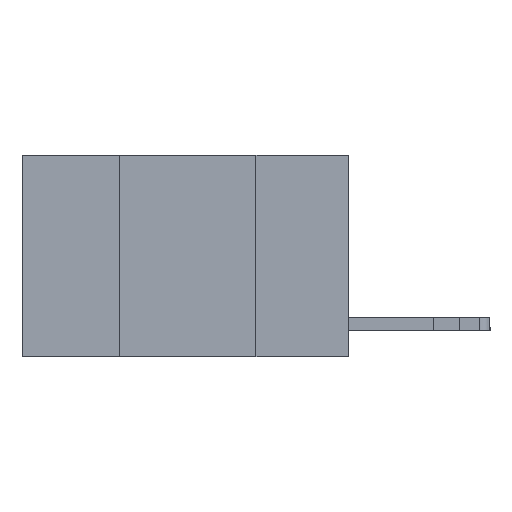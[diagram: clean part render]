
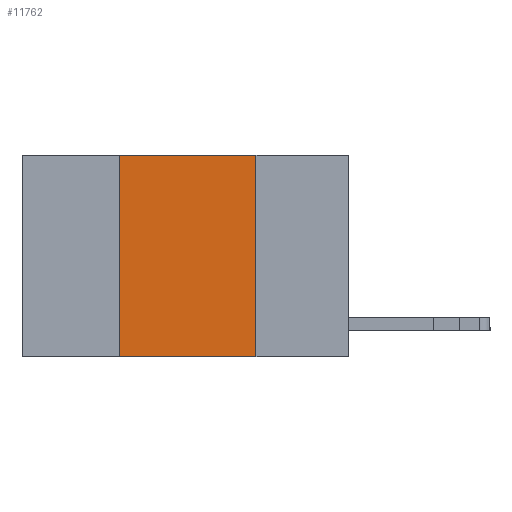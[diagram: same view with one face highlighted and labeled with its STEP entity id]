
A CAD part, left-side view. The second image highlights one B-rep face of the part: STEP entity #11762.
In plain terms, the highlighted planar face has unit normal (-1, 0, 0).
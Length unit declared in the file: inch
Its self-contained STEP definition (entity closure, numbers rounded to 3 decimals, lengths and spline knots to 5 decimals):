
#1305 = DIRECTION ( 'NONE',  ( 0., 0., -1. ) ) ;
#2176 = DIRECTION ( 'NONE',  ( 0., -1., 0. ) ) ;
#2250 = VERTEX_POINT ( 'NONE', #21121 ) ;
#2706 = EDGE_CURVE ( 'NONE', #9920, #2250, #7418, .T. ) ;
#3280 = LINE ( 'NONE', #18351, #7762 ) ;
#3297 = ORIENTED_EDGE ( 'NONE', *, *, #14448, .F. ) ;
#3431 = ORIENTED_EDGE ( 'NONE', *, *, #2706, .F. ) ;
#3843 = LINE ( 'NONE', #17492, #4286 ) ;
#3844 = EDGE_CURVE ( 'NONE', #9920, #5923, #13802, .T. ) ;
#3925 = CARTESIAN_POINT ( 'NONE',  ( 0., 0.6, -0.37 ) ) ;
#4168 = DIRECTION ( 'NONE',  ( 0., 0., -1. ) ) ;
#4286 = VECTOR ( 'NONE', #15497, 39.37008 ) ;
#5923 = VERTEX_POINT ( 'NONE', #7495 ) ;
#5963 = AXIS2_PLACEMENT_3D ( 'NONE', #14273, #17820, #4168 ) ;
#7418 = LINE ( 'NONE', #21324, #15667 ) ;
#7495 = CARTESIAN_POINT ( 'NONE',  ( 0., 0.17, -0.37 ) ) ;
#7762 = VECTOR ( 'NONE', #1305, 39.37008 ) ;
#8554 = EDGE_LOOP ( 'NONE', ( #3297, #17894, #3431, #17116 ) ) ;
#9545 = VECTOR ( 'NONE', #2176, 39.37008 ) ;
#9920 = VERTEX_POINT ( 'NONE', #21531 ) ;
#11762 = ADVANCED_FACE ( 'NONE', ( #12742 ), #14160, .F. ) ;
#12742 = FACE_OUTER_BOUND ( 'NONE', #8554, .T. ) ;
#13500 = CARTESIAN_POINT ( 'NONE',  ( 0., 0.17, 0. ) ) ;
#13802 = LINE ( 'NONE', #3925, #9545 ) ;
#14122 = DIRECTION ( 'NONE',  ( 0., 0., 1. ) ) ;
#14160 = PLANE ( 'NONE',  #5963 ) ;
#14273 = CARTESIAN_POINT ( 'NONE',  ( 0., 0.6, 0. ) ) ;
#14448 = EDGE_CURVE ( 'NONE', #15435, #5923, #3280, .T. ) ;
#15435 = VERTEX_POINT ( 'NONE', #13500 ) ;
#15497 = DIRECTION ( 'NONE',  ( 0., -1., 0. ) ) ;
#15667 = VECTOR ( 'NONE', #14122, 39.37008 ) ;
#16860 = EDGE_CURVE ( 'NONE', #2250, #15435, #3843, .T. ) ;
#17116 = ORIENTED_EDGE ( 'NONE', *, *, #3844, .T. ) ;
#17492 = CARTESIAN_POINT ( 'NONE',  ( 0., 0.6, 0. ) ) ;
#17820 = DIRECTION ( 'NONE',  ( 1., 0., 0. ) ) ;
#17894 = ORIENTED_EDGE ( 'NONE', *, *, #16860, .F. ) ;
#18351 = CARTESIAN_POINT ( 'NONE',  ( 0., 0.17, 0. ) ) ;
#21121 = CARTESIAN_POINT ( 'NONE',  ( 0., 0.42, 0. ) ) ;
#21324 = CARTESIAN_POINT ( 'NONE',  ( 0., 0.42, 0. ) ) ;
#21531 = CARTESIAN_POINT ( 'NONE',  ( 0., 0.42, -0.37 ) ) ;
